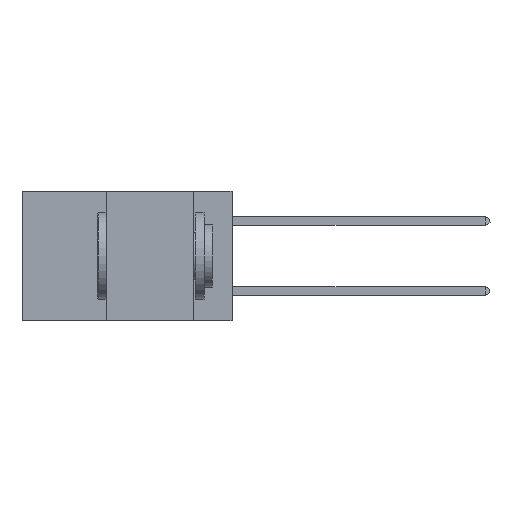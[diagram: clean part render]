
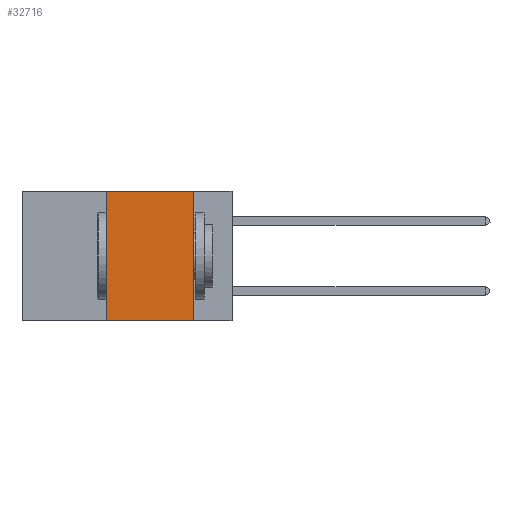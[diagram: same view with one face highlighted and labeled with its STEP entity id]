
A CAD part, left-side view. The second image highlights one B-rep face of the part: STEP entity #32716.
In plain terms, the highlighted planar face has unit normal (-1, 0, 0).
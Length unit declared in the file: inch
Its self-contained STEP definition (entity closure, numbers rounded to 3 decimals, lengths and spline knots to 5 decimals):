
#188 = VERTEX_POINT ( 'NONE', #8033 ) ;
#1555 = DIRECTION ( 'NONE',  ( 0., -1., 0. ) ) ;
#4258 = CARTESIAN_POINT ( 'NONE',  ( 0., 0.6, 0. ) ) ;
#6109 = PLANE ( 'NONE',  #24073 ) ;
#6457 = DIRECTION ( 'NONE',  ( 1., 0., 0. ) ) ;
#6929 = CARTESIAN_POINT ( 'NONE',  ( 0., 0.36, 0. ) ) ;
#7684 = CARTESIAN_POINT ( 'NONE',  ( 0., 0.36, -0.37 ) ) ;
#8033 = CARTESIAN_POINT ( 'NONE',  ( 0., 0.36, 0. ) ) ;
#8866 = ORIENTED_EDGE ( 'NONE', *, *, #25100, .F. ) ;
#10254 = EDGE_CURVE ( 'NONE', #188, #16264, #16081, .T. ) ;
#11699 = DIRECTION ( 'NONE',  ( 0., -1., 0. ) ) ;
#11892 = VERTEX_POINT ( 'NONE', #36141 ) ;
#13044 = EDGE_CURVE ( 'NONE', #29561, #11892, #22520, .T. ) ;
#13383 = CARTESIAN_POINT ( 'NONE',  ( 0., 0.6, -0.37 ) ) ;
#13716 = EDGE_CURVE ( 'NONE', #29561, #188, #14050, .T. ) ;
#14050 = LINE ( 'NONE', #6929, #22490 ) ;
#15146 = DIRECTION ( 'NONE',  ( 0., 0., 1. ) ) ;
#15406 = VECTOR ( 'NONE', #1555, 39.37008 ) ;
#16081 = LINE ( 'NONE', #4258, #22753 ) ;
#16264 = VERTEX_POINT ( 'NONE', #19227 ) ;
#18065 = EDGE_LOOP ( 'NONE', ( #8866, #30856, #33238, #24579 ) ) ;
#19227 = CARTESIAN_POINT ( 'NONE',  ( 0., 0.11, 0. ) ) ;
#20494 = DIRECTION ( 'NONE',  ( 0., 0., -1. ) ) ;
#21079 = DIRECTION ( 'NONE',  ( 0., 0., -1. ) ) ;
#22490 = VECTOR ( 'NONE', #15146, 39.37008 ) ;
#22520 = LINE ( 'NONE', #13383, #15406 ) ;
#22753 = VECTOR ( 'NONE', #11699, 39.37008 ) ;
#23442 = CARTESIAN_POINT ( 'NONE',  ( 0., 0.6, 0. ) ) ;
#24073 = AXIS2_PLACEMENT_3D ( 'NONE', #23442, #6457, #20494 ) ;
#24579 = ORIENTED_EDGE ( 'NONE', *, *, #13044, .T. ) ;
#25100 = EDGE_CURVE ( 'NONE', #16264, #11892, #33157, .T. ) ;
#29317 = CARTESIAN_POINT ( 'NONE',  ( 0., 0.11, 0. ) ) ;
#29561 = VERTEX_POINT ( 'NONE', #7684 ) ;
#30856 = ORIENTED_EDGE ( 'NONE', *, *, #10254, .F. ) ;
#32716 = ADVANCED_FACE ( 'NONE', ( #33113 ), #6109, .F. ) ;
#33113 = FACE_OUTER_BOUND ( 'NONE', #18065, .T. ) ;
#33157 = LINE ( 'NONE', #29317, #33618 ) ;
#33238 = ORIENTED_EDGE ( 'NONE', *, *, #13716, .F. ) ;
#33618 = VECTOR ( 'NONE', #21079, 39.37008 ) ;
#36141 = CARTESIAN_POINT ( 'NONE',  ( 0., 0.11, -0.37 ) ) ;
